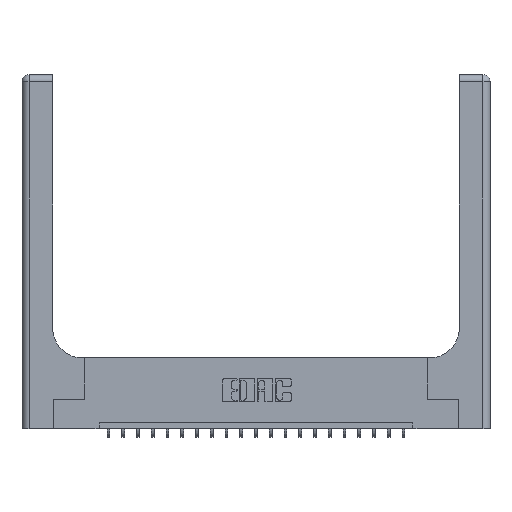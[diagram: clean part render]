
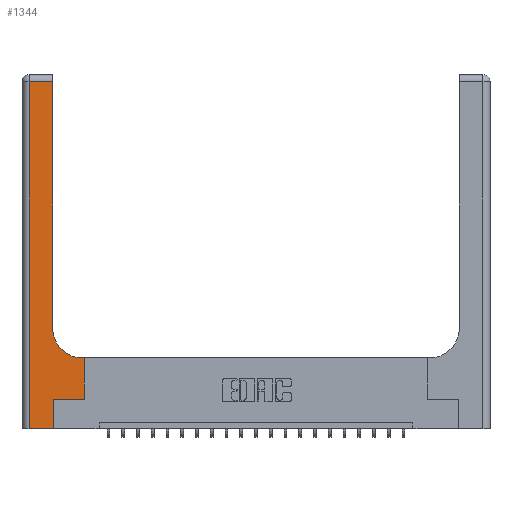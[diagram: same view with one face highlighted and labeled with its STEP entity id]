
A CAD part, top view. The second image highlights one B-rep face of the part: STEP entity #1344.
In plain terms, the highlighted planar face has unit normal (0, 0, 1).
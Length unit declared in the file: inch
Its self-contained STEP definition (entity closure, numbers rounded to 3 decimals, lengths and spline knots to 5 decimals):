
#196 = EDGE_CURVE ( 'NONE', #19925, #19410, #21477, .T. ) ;
#221 = DIRECTION ( 'NONE',  ( 0., 0., -1. ) ) ;
#288 = VERTEX_POINT ( 'NONE', #6534 ) ;
#452 = AXIS2_PLACEMENT_3D ( 'NONE', #4174, #15950, #1023 ) ;
#683 = VERTEX_POINT ( 'NONE', #6840 ) ;
#814 = LINE ( 'NONE', #11059, #3722 ) ;
#1023 = DIRECTION ( 'NONE',  ( -1., 0., 0. ) ) ;
#1344 = ADVANCED_FACE ( 'NONE', ( #14191 ), #2328, .F. ) ;
#1757 = CARTESIAN_POINT ( 'NONE',  ( 0.51, 0.85, 0.37 ) ) ;
#1781 = CARTESIAN_POINT ( 'NONE',  ( 0.26, 0.85, 0.37 ) ) ;
#2328 = PLANE ( 'NONE',  #452 ) ;
#2517 = ORIENTED_EDGE ( 'NONE', *, *, #196, .T. ) ;
#2809 = CARTESIAN_POINT ( 'NONE',  ( 0.528, 0.25, 0.37 ) ) ;
#2820 = EDGE_LOOP ( 'NONE', ( #9419, #20693, #2517, #9139, #14459, #18671, #17102, #8624, #5733 ) ) ;
#3276 = CARTESIAN_POINT ( 'NONE',  ( 0.06, 2.94, 0.37 ) ) ;
#3418 = DIRECTION ( 'NONE',  ( -1., 0., 0. ) ) ;
#3722 = VECTOR ( 'NONE', #19023, 39.37008 ) ;
#3875 = LINE ( 'NONE', #20133, #5026 ) ;
#3979 = CARTESIAN_POINT ( 'NONE',  ( 0.528, 0.6, 0.37 ) ) ;
#4174 = CARTESIAN_POINT ( 'NONE',  ( 0., 3., 0.37 ) ) ;
#4184 = CARTESIAN_POINT ( 'NONE',  ( 0.06, 0., 0.37 ) ) ;
#4870 = EDGE_CURVE ( 'NONE', #19305, #5889, #3875, .T. ) ;
#5012 = DIRECTION ( 'NONE',  ( 0., -1., 0. ) ) ;
#5026 = VECTOR ( 'NONE', #12271, 39.37008 ) ;
#5733 = ORIENTED_EDGE ( 'NONE', *, *, #16820, .T. ) ;
#5884 = LINE ( 'NONE', #14050, #14697 ) ;
#5886 = VECTOR ( 'NONE', #17898, 39.37008 ) ;
#5889 = VERTEX_POINT ( 'NONE', #12721 ) ;
#6020 = LINE ( 'NONE', #9513, #5886 ) ;
#6155 = DIRECTION ( 'NONE',  ( 1., 0., 0. ) ) ;
#6377 = LINE ( 'NONE', #21100, #19120 ) ;
#6534 = CARTESIAN_POINT ( 'NONE',  ( 0.265, 0., 0.37 ) ) ;
#6840 = CARTESIAN_POINT ( 'NONE',  ( 0.26, 2.94, 0.37 ) ) ;
#7881 = EDGE_CURVE ( 'NONE', #20874, #683, #814, .T. ) ;
#8624 = ORIENTED_EDGE ( 'NONE', *, *, #4870, .T. ) ;
#9139 = ORIENTED_EDGE ( 'NONE', *, *, #12593, .T. ) ;
#9224 = LINE ( 'NONE', #12717, #14783 ) ;
#9419 = ORIENTED_EDGE ( 'NONE', *, *, #7881, .T. ) ;
#9513 = CARTESIAN_POINT ( 'NONE',  ( 0., 0., 0.37 ) ) ;
#9934 = DIRECTION ( 'NONE',  ( 1., 0., 0. ) ) ;
#11059 = CARTESIAN_POINT ( 'NONE',  ( 0.26, 3., 0.37 ) ) ;
#11243 = VECTOR ( 'NONE', #3418, 39.37008 ) ;
#11709 = LINE ( 'NONE', #18347, #11243 ) ;
#12066 = EDGE_CURVE ( 'NONE', #18220, #18746, #6377, .T. ) ;
#12271 = DIRECTION ( 'NONE',  ( -1., 0., 0. ) ) ;
#12593 = EDGE_CURVE ( 'NONE', #19410, #288, #6020, .T. ) ;
#12717 = CARTESIAN_POINT ( 'NONE',  ( 0.265, 0., 0.37 ) ) ;
#12721 = CARTESIAN_POINT ( 'NONE',  ( 0.51, 0.6, 0.37 ) ) ;
#14050 = CARTESIAN_POINT ( 'NONE',  ( 0.528, 0.25, 0.37 ) ) ;
#14191 = FACE_OUTER_BOUND ( 'NONE', #2820, .T. ) ;
#14459 = ORIENTED_EDGE ( 'NONE', *, *, #20137, .T. ) ;
#14677 = AXIS2_PLACEMENT_3D ( 'NONE', #1757, #221, #9934 ) ;
#14697 = VECTOR ( 'NONE', #20495, 39.37008 ) ;
#14783 = VECTOR ( 'NONE', #17838, 39.37008 ) ;
#15950 = DIRECTION ( 'NONE',  ( 0., 0., -1. ) ) ;
#16351 = CARTESIAN_POINT ( 'NONE',  ( 0.06, 3., 0.37 ) ) ;
#16820 = EDGE_CURVE ( 'NONE', #5889, #20874, #18514, .T. ) ;
#16997 = EDGE_CURVE ( 'NONE', #18746, #19305, #5884, .T. ) ;
#17102 = ORIENTED_EDGE ( 'NONE', *, *, #16997, .T. ) ;
#17606 = EDGE_CURVE ( 'NONE', #683, #19925, #11709, .T. ) ;
#17838 = DIRECTION ( 'NONE',  ( 0., 1., 0. ) ) ;
#17898 = DIRECTION ( 'NONE',  ( 1., 0., 0. ) ) ;
#18220 = VERTEX_POINT ( 'NONE', #20620 ) ;
#18347 = CARTESIAN_POINT ( 'NONE',  ( 0., 2.94, 0.37 ) ) ;
#18514 = CIRCLE ( 'NONE', #14677, 0.25 ) ;
#18671 = ORIENTED_EDGE ( 'NONE', *, *, #12066, .T. ) ;
#18746 = VERTEX_POINT ( 'NONE', #2809 ) ;
#19023 = DIRECTION ( 'NONE',  ( 0., 1., 0. ) ) ;
#19120 = VECTOR ( 'NONE', #6155, 39.37008 ) ;
#19140 = VECTOR ( 'NONE', #5012, 39.37008 ) ;
#19305 = VERTEX_POINT ( 'NONE', #3979 ) ;
#19410 = VERTEX_POINT ( 'NONE', #4184 ) ;
#19925 = VERTEX_POINT ( 'NONE', #3276 ) ;
#20133 = CARTESIAN_POINT ( 'NONE',  ( 0.26, 0.6, 0.37 ) ) ;
#20137 = EDGE_CURVE ( 'NONE', #288, #18220, #9224, .T. ) ;
#20495 = DIRECTION ( 'NONE',  ( 0., 1., 0. ) ) ;
#20620 = CARTESIAN_POINT ( 'NONE',  ( 0.265, 0.25, 0.37 ) ) ;
#20693 = ORIENTED_EDGE ( 'NONE', *, *, #17606, .T. ) ;
#20874 = VERTEX_POINT ( 'NONE', #1781 ) ;
#21100 = CARTESIAN_POINT ( 'NONE',  ( 0.265, 0.25, 0.37 ) ) ;
#21477 = LINE ( 'NONE', #16351, #19140 ) ;
